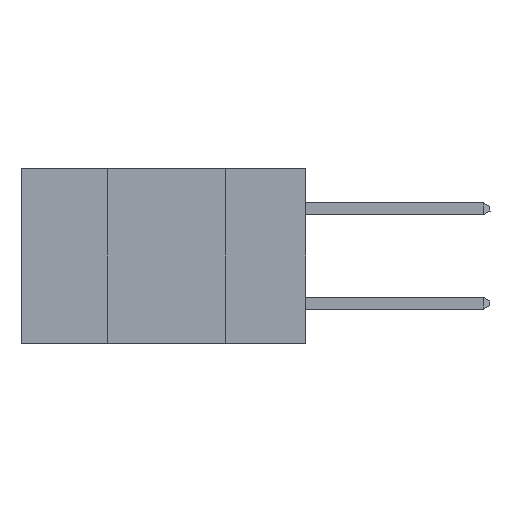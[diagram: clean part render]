
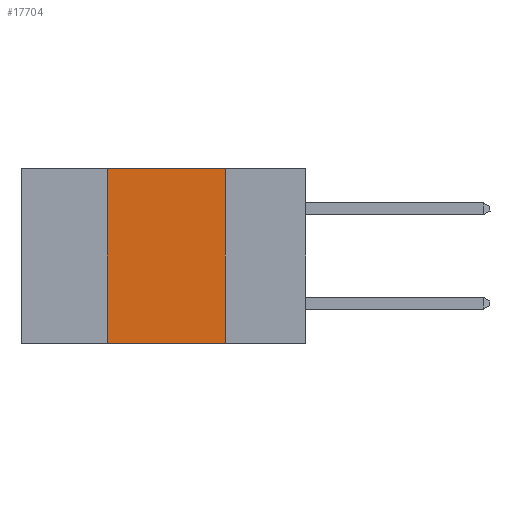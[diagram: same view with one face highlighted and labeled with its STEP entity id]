
A CAD part, left-side view. The second image highlights one B-rep face of the part: STEP entity #17704.
In plain terms, the highlighted planar face has unit normal (-1, 0, 0).
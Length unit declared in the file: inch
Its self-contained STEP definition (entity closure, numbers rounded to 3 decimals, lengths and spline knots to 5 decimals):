
#438 = PLANE ( 'NONE',  #8100 ) ;
#516 = VECTOR ( 'NONE', #24636, 39.37008 ) ;
#693 = EDGE_CURVE ( 'NONE', #20132, #12419, #2033, .T. ) ;
#1198 = CARTESIAN_POINT ( 'NONE',  ( 0., 0.42, -0.37 ) ) ;
#2033 = LINE ( 'NONE', #9177, #17833 ) ;
#3568 = ORIENTED_EDGE ( 'NONE', *, *, #17301, .F. ) ;
#4755 = ORIENTED_EDGE ( 'NONE', *, *, #693, .F. ) ;
#5581 = CARTESIAN_POINT ( 'NONE',  ( 0., 0.17, -0.37 ) ) ;
#5693 = LINE ( 'NONE', #23019, #8484 ) ;
#6356 = ORIENTED_EDGE ( 'NONE', *, *, #12683, .F. ) ;
#7503 = DIRECTION ( 'NONE',  ( 0., -1., 0. ) ) ;
#8100 = AXIS2_PLACEMENT_3D ( 'NONE', #8107, #8450, #22327 ) ;
#8107 = CARTESIAN_POINT ( 'NONE',  ( 0., 0.6, 0. ) ) ;
#8450 = DIRECTION ( 'NONE',  ( 1., 0., 0. ) ) ;
#8484 = VECTOR ( 'NONE', #7503, 39.37008 ) ;
#9177 = CARTESIAN_POINT ( 'NONE',  ( 0., 0.6, 0. ) ) ;
#9852 = CARTESIAN_POINT ( 'NONE',  ( 0., 0.17, 0. ) ) ;
#10484 = CARTESIAN_POINT ( 'NONE',  ( 0., 0.42, 0. ) ) ;
#11011 = DIRECTION ( 'NONE',  ( 0., 0., -1. ) ) ;
#12419 = VERTEX_POINT ( 'NONE', #9852 ) ;
#12683 = EDGE_CURVE ( 'NONE', #15637, #20132, #13206, .T. ) ;
#12714 = CARTESIAN_POINT ( 'NONE',  ( 0., 0.42, 0. ) ) ;
#12932 = VECTOR ( 'NONE', #11011, 39.37008 ) ;
#13206 = LINE ( 'NONE', #12714, #516 ) ;
#13574 = LINE ( 'NONE', #18890, #12932 ) ;
#13873 = FACE_OUTER_BOUND ( 'NONE', #20732, .T. ) ;
#14769 = DIRECTION ( 'NONE',  ( 0., -1., 0. ) ) ;
#15637 = VERTEX_POINT ( 'NONE', #1198 ) ;
#17301 = EDGE_CURVE ( 'NONE', #12419, #19914, #13574, .T. ) ;
#17704 = ADVANCED_FACE ( 'NONE', ( #13873 ), #438, .F. ) ;
#17833 = VECTOR ( 'NONE', #14769, 39.37008 ) ;
#18890 = CARTESIAN_POINT ( 'NONE',  ( 0., 0.17, 0. ) ) ;
#19324 = EDGE_CURVE ( 'NONE', #15637, #19914, #5693, .T. ) ;
#19914 = VERTEX_POINT ( 'NONE', #5581 ) ;
#20132 = VERTEX_POINT ( 'NONE', #10484 ) ;
#20732 = EDGE_LOOP ( 'NONE', ( #3568, #4755, #6356, #22464 ) ) ;
#22327 = DIRECTION ( 'NONE',  ( 0., 0., -1. ) ) ;
#22464 = ORIENTED_EDGE ( 'NONE', *, *, #19324, .T. ) ;
#23019 = CARTESIAN_POINT ( 'NONE',  ( 0., 0.6, -0.37 ) ) ;
#24636 = DIRECTION ( 'NONE',  ( 0., 0., 1. ) ) ;
